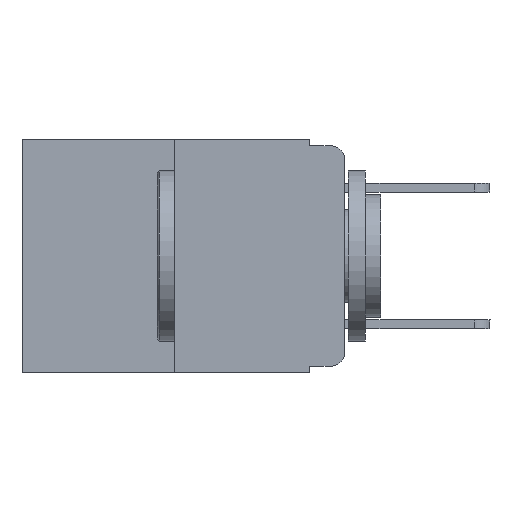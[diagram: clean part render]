
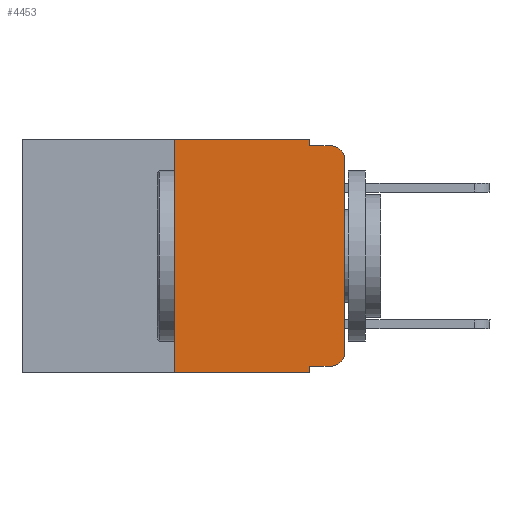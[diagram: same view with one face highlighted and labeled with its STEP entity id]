
A CAD part, left-side view. The second image highlights one B-rep face of the part: STEP entity #4453.
In plain terms, the highlighted planar face has unit normal (-1, 0, 0).
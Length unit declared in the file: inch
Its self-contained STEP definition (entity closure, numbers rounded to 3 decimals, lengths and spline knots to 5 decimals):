
#39 = VECTOR ( 'NONE', #10454, 39.37008 ) ;
#664 = EDGE_CURVE ( 'NONE', #5747, #1337, #13942, .T. ) ;
#828 = CARTESIAN_POINT ( 'NONE',  ( 0., 0.051, -0.333 ) ) ;
#1137 = VECTOR ( 'NONE', #15797, 39.37008 ) ;
#1337 = VERTEX_POINT ( 'NONE', #11348 ) ;
#1737 = CARTESIAN_POINT ( 'NONE',  ( 0., 0.051, -0.333 ) ) ;
#2094 = CARTESIAN_POINT ( 'NONE',  ( 0., 0.051, 0. ) ) ;
#2705 = CARTESIAN_POINT ( 'NONE',  ( 0., 0.051, 0. ) ) ;
#3037 = LINE ( 'NONE', #8550, #39 ) ;
#3092 = DIRECTION ( 'NONE',  ( 0., -1., 0. ) ) ;
#3663 = DIRECTION ( 'NONE',  ( 0., -1., 0. ) ) ;
#3722 = DIRECTION ( 'NONE',  ( 0., 0., -1. ) ) ;
#3822 = ORIENTED_EDGE ( 'NONE', *, *, #8331, .T. ) ;
#3831 = VECTOR ( 'NONE', #3663, 39.37008 ) ;
#3841 = CARTESIAN_POINT ( 'NONE',  ( 0., 0., 0. ) ) ;
#3900 = VERTEX_POINT ( 'NONE', #14265 ) ;
#3951 = DIRECTION ( 'NONE',  ( 1., 0., 0. ) ) ;
#4021 = DIRECTION ( 'NONE',  ( 0., 0., -1. ) ) ;
#4048 = ORIENTED_EDGE ( 'NONE', *, *, #5423, .F. ) ;
#4347 = LINE ( 'NONE', #3841, #22473 ) ;
#4453 = ADVANCED_FACE ( 'NONE', ( #14954 ), #13396, .F. ) ;
#5082 = LINE ( 'NONE', #9451, #19668 ) ;
#5265 = VERTEX_POINT ( 'NONE', #19562 ) ;
#5423 = EDGE_CURVE ( 'NONE', #3900, #18782, #3037, .T. ) ;
#5616 = CIRCLE ( 'NONE', #23873, 0.02 ) ;
#5655 = ORIENTED_EDGE ( 'NONE', *, *, #7094, .F. ) ;
#5747 = VERTEX_POINT ( 'NONE', #12947 ) ;
#6580 = LINE ( 'NONE', #2094, #9547 ) ;
#7094 = EDGE_CURVE ( 'NONE', #18782, #7933, #6580, .T. ) ;
#7505 = EDGE_CURVE ( 'NONE', #7960, #1337, #5082, .T. ) ;
#7731 = EDGE_CURVE ( 'NONE', #5747, #3900, #19358, .T. ) ;
#7733 = CARTESIAN_POINT ( 'NONE',  ( 0., 0.02, -0.03 ) ) ;
#7933 = VERTEX_POINT ( 'NONE', #8294 ) ;
#7960 = VERTEX_POINT ( 'NONE', #828 ) ;
#8091 = EDGE_LOOP ( 'NONE', ( #12038, #3822, #15866, #5655, #4048, #14368, #16088, #11984, #21380, #10252 ) ) ;
#8294 = CARTESIAN_POINT ( 'NONE',  ( 0., 0.051, -0.01 ) ) ;
#8331 = EDGE_CURVE ( 'NONE', #15716, #15820, #5616, .T. ) ;
#8550 = CARTESIAN_POINT ( 'NONE',  ( 0., 0.473, 0. ) ) ;
#9446 = LINE ( 'NONE', #21960, #18088 ) ;
#9451 = CARTESIAN_POINT ( 'NONE',  ( 0., 0.051, 0. ) ) ;
#9547 = VECTOR ( 'NONE', #3722, 39.37008 ) ;
#10090 = VECTOR ( 'NONE', #17030, 39.37008 ) ;
#10252 = ORIENTED_EDGE ( 'NONE', *, *, #17636, .T. ) ;
#10454 = DIRECTION ( 'NONE',  ( 0., -1., 0. ) ) ;
#10521 = EDGE_CURVE ( 'NONE', #20635, #15716, #4347, .T. ) ;
#10813 = DIRECTION ( 'NONE',  ( -1., 0., 0. ) ) ;
#10977 = CARTESIAN_POINT ( 'NONE',  ( 0., 0.02, -0.313 ) ) ;
#11348 = CARTESIAN_POINT ( 'NONE',  ( 0., 0.051, -0.343 ) ) ;
#11478 = CARTESIAN_POINT ( 'NONE',  ( 0., 0.25, 0. ) ) ;
#11984 = ORIENTED_EDGE ( 'NONE', *, *, #7505, .F. ) ;
#12038 = ORIENTED_EDGE ( 'NONE', *, *, #10521, .T. ) ;
#12947 = CARTESIAN_POINT ( 'NONE',  ( 0., 0.25, -0.343 ) ) ;
#13396 = PLANE ( 'NONE',  #21705 ) ;
#13562 = DIRECTION ( 'NONE',  ( -1., 0., 0. ) ) ;
#13942 = LINE ( 'NONE', #15885, #1137 ) ;
#14265 = CARTESIAN_POINT ( 'NONE',  ( 0., 0.25, 0. ) ) ;
#14368 = ORIENTED_EDGE ( 'NONE', *, *, #7731, .F. ) ;
#14954 = FACE_OUTER_BOUND ( 'NONE', #8091, .T. ) ;
#15302 = CARTESIAN_POINT ( 'NONE',  ( 0., 0.473, 0. ) ) ;
#15650 = CARTESIAN_POINT ( 'NONE',  ( 0., 0., -0.03 ) ) ;
#15716 = VERTEX_POINT ( 'NONE', #15650 ) ;
#15797 = DIRECTION ( 'NONE',  ( 0., -1., 0. ) ) ;
#15820 = VERTEX_POINT ( 'NONE', #23590 ) ;
#15866 = ORIENTED_EDGE ( 'NONE', *, *, #18162, .F. ) ;
#15885 = CARTESIAN_POINT ( 'NONE',  ( 0., 0.473, -0.343 ) ) ;
#16088 = ORIENTED_EDGE ( 'NONE', *, *, #664, .T. ) ;
#16756 = AXIS2_PLACEMENT_3D ( 'NONE', #10977, #10813, #24207 ) ;
#17030 = DIRECTION ( 'NONE',  ( 0., 0., 1. ) ) ;
#17115 = CARTESIAN_POINT ( 'NONE',  ( 0., 0., -0.313 ) ) ;
#17208 = DIRECTION ( 'NONE',  ( 0., 0., -1. ) ) ;
#17636 = EDGE_CURVE ( 'NONE', #5265, #20635, #19023, .T. ) ;
#18088 = VECTOR ( 'NONE', #3092, 39.37008 ) ;
#18162 = EDGE_CURVE ( 'NONE', #7933, #15820, #9446, .T. ) ;
#18358 = EDGE_CURVE ( 'NONE', #7960, #5265, #24036, .T. ) ;
#18782 = VERTEX_POINT ( 'NONE', #2705 ) ;
#19023 = CIRCLE ( 'NONE', #16756, 0.02 ) ;
#19358 = LINE ( 'NONE', #11478, #10090 ) ;
#19562 = CARTESIAN_POINT ( 'NONE',  ( 0., 0.02, -0.333 ) ) ;
#19668 = VECTOR ( 'NONE', #22756, 39.37008 ) ;
#20635 = VERTEX_POINT ( 'NONE', #17115 ) ;
#21380 = ORIENTED_EDGE ( 'NONE', *, *, #18358, .T. ) ;
#21705 = AXIS2_PLACEMENT_3D ( 'NONE', #15302, #3951, #17208 ) ;
#21960 = CARTESIAN_POINT ( 'NONE',  ( 0., 0.051, -0.01 ) ) ;
#22473 = VECTOR ( 'NONE', #22594, 39.37008 ) ;
#22594 = DIRECTION ( 'NONE',  ( 0., 0., 1. ) ) ;
#22756 = DIRECTION ( 'NONE',  ( 0., 0., -1. ) ) ;
#23590 = CARTESIAN_POINT ( 'NONE',  ( 0., 0.02, -0.01 ) ) ;
#23873 = AXIS2_PLACEMENT_3D ( 'NONE', #7733, #13562, #4021 ) ;
#24036 = LINE ( 'NONE', #1737, #3831 ) ;
#24207 = DIRECTION ( 'NONE',  ( 0., 0., -1. ) ) ;
